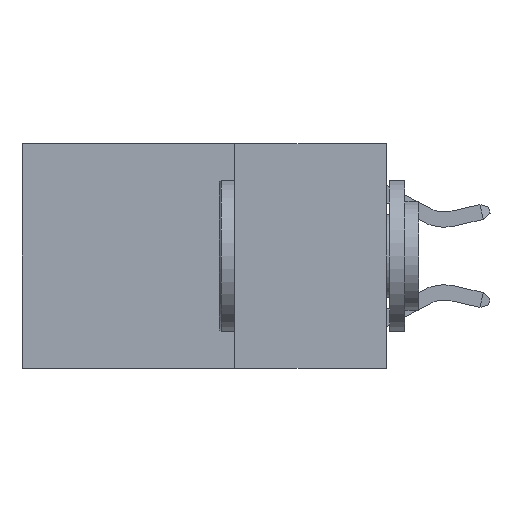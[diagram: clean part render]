
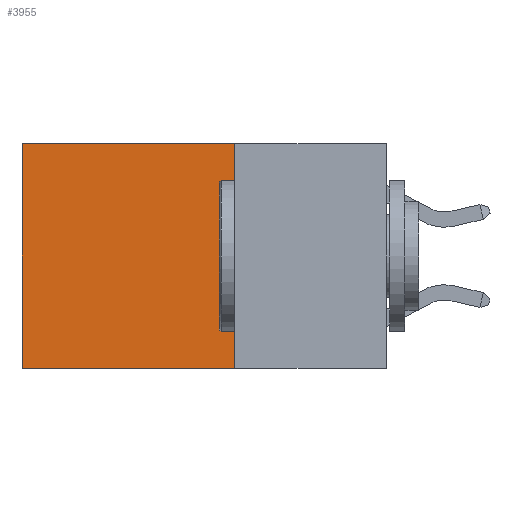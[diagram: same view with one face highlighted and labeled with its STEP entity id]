
A CAD part, left-side view. The second image highlights one B-rep face of the part: STEP entity #3955.
In plain terms, the highlighted planar face has unit normal (-1, 0, 0).
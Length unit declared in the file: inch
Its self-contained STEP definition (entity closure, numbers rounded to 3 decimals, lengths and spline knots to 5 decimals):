
#2178 = AXIS2_PLACEMENT_3D ( 'NONE', #15380, #24055, #7990 ) ;
#2915 = DIRECTION ( 'NONE',  ( 0., 1., 0. ) ) ;
#3205 = LINE ( 'NONE', #20760, #11668 ) ;
#3265 = VECTOR ( 'NONE', #23185, 39.37008 ) ;
#3955 = ADVANCED_FACE ( 'NONE', ( #13366 ), #6628, .F. ) ;
#5441 = EDGE_CURVE ( 'NONE', #11805, #7827, #3205, .T. ) ;
#6156 = LINE ( 'NONE', #28023, #3265 ) ;
#6552 = ORIENTED_EDGE ( 'NONE', *, *, #5441, .T. ) ;
#6628 = PLANE ( 'NONE',  #2178 ) ;
#7827 = VERTEX_POINT ( 'NONE', #8714 ) ;
#7990 = DIRECTION ( 'NONE',  ( 0., 0., -1. ) ) ;
#8714 = CARTESIAN_POINT ( 'NONE',  ( 0.2625, 0.6, 0. ) ) ;
#8731 = LINE ( 'NONE', #11438, #20707 ) ;
#9150 = DIRECTION ( 'NONE',  ( 0., 0., -1. ) ) ;
#9997 = CARTESIAN_POINT ( 'NONE',  ( 0.2625, 0.25, -0.37 ) ) ;
#11438 = CARTESIAN_POINT ( 'NONE',  ( 0.2625, 0.6, 0. ) ) ;
#11668 = VECTOR ( 'NONE', #2915, 39.37008 ) ;
#11805 = VERTEX_POINT ( 'NONE', #21034 ) ;
#12061 = CARTESIAN_POINT ( 'NONE',  ( 0.2625, 0.6, -0.37 ) ) ;
#12498 = VERTEX_POINT ( 'NONE', #12061 ) ;
#13265 = EDGE_CURVE ( 'NONE', #7827, #12498, #8731, .T. ) ;
#13366 = FACE_OUTER_BOUND ( 'NONE', #16262, .T. ) ;
#13921 = VERTEX_POINT ( 'NONE', #25186 ) ;
#15380 = CARTESIAN_POINT ( 'NONE',  ( 0.2625, 0.25, 0. ) ) ;
#16159 = ORIENTED_EDGE ( 'NONE', *, *, #27684, .F. ) ;
#16262 = EDGE_LOOP ( 'NONE', ( #20332, #18239, #16159, #6552 ) ) ;
#16795 = VECTOR ( 'NONE', #18706, 39.37008 ) ;
#18239 = ORIENTED_EDGE ( 'NONE', *, *, #24038, .F. ) ;
#18706 = DIRECTION ( 'NONE',  ( 0., 1., 0. ) ) ;
#20332 = ORIENTED_EDGE ( 'NONE', *, *, #13265, .T. ) ;
#20707 = VECTOR ( 'NONE', #9150, 39.37008 ) ;
#20760 = CARTESIAN_POINT ( 'NONE',  ( 0.2625, 0.25, 0. ) ) ;
#21034 = CARTESIAN_POINT ( 'NONE',  ( 0.2625, 0.25, 0. ) ) ;
#23185 = DIRECTION ( 'NONE',  ( 0., 0., -1. ) ) ;
#24038 = EDGE_CURVE ( 'NONE', #13921, #12498, #25115, .T. ) ;
#24055 = DIRECTION ( 'NONE',  ( 1., 0., 0. ) ) ;
#25115 = LINE ( 'NONE', #9997, #16795 ) ;
#25186 = CARTESIAN_POINT ( 'NONE',  ( 0.2625, 0.25, -0.37 ) ) ;
#27684 = EDGE_CURVE ( 'NONE', #11805, #13921, #6156, .T. ) ;
#28023 = CARTESIAN_POINT ( 'NONE',  ( 0.2625, 0.25, 0. ) ) ;
